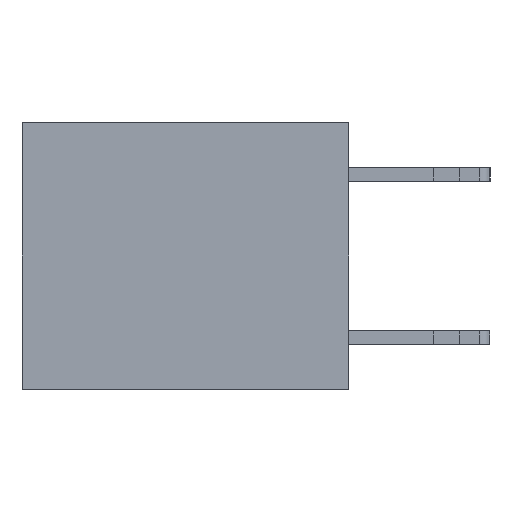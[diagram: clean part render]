
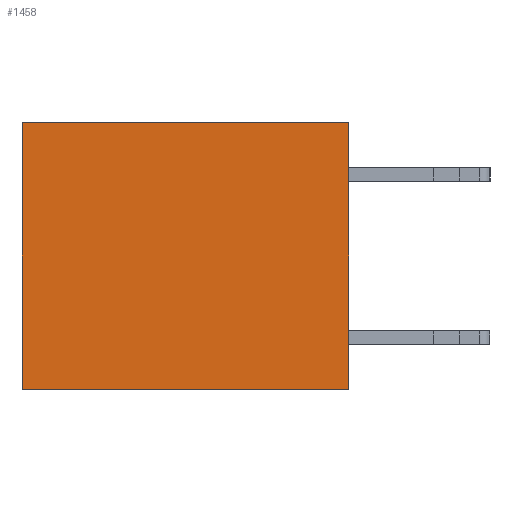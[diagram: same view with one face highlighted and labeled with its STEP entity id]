
A CAD part, left-side view. The second image highlights one B-rep face of the part: STEP entity #1458.
In plain terms, the highlighted planar face has unit normal (-1, 0, 0).
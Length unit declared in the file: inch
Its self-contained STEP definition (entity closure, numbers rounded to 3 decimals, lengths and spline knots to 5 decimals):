
#88 = ORIENTED_EDGE ( 'NONE', *, *, #11101, .T. ) ;
#96 = LINE ( 'NONE', #9933, #14800 ) ;
#450 = CARTESIAN_POINT ( 'NONE',  ( 0.3165, 0., 0. ) ) ;
#704 = VERTEX_POINT ( 'NONE', #18247 ) ;
#1458 = ADVANCED_FACE ( 'NONE', ( #15243 ), #18003, .F. ) ;
#2218 = AXIS2_PLACEMENT_3D ( 'NONE', #15051, #9306, #4893 ) ;
#3827 = LINE ( 'NONE', #7622, #7170 ) ;
#4893 = DIRECTION ( 'NONE',  ( 0., 0., -1. ) ) ;
#4894 = CARTESIAN_POINT ( 'NONE',  ( 0.3165, 0., -0.49 ) ) ;
#5191 = VERTEX_POINT ( 'NONE', #5452 ) ;
#5337 = EDGE_CURVE ( 'NONE', #12923, #704, #9621, .T. ) ;
#5452 = CARTESIAN_POINT ( 'NONE',  ( 0.3165, 0., -0.49 ) ) ;
#7170 = VECTOR ( 'NONE', #17742, 39.37008 ) ;
#7622 = CARTESIAN_POINT ( 'NONE',  ( 0.3165, 0., -0.49 ) ) ;
#7846 = ORIENTED_EDGE ( 'NONE', *, *, #13247, .F. ) ;
#8330 = EDGE_CURVE ( 'NONE', #5191, #14550, #11269, .T. ) ;
#9306 = DIRECTION ( 'NONE',  ( 1., 0., 0. ) ) ;
#9621 = LINE ( 'NONE', #12987, #15422 ) ;
#9926 = DIRECTION ( 'NONE',  ( 0., 1., 0. ) ) ;
#9933 = CARTESIAN_POINT ( 'NONE',  ( 0.3165, 0.6, -0.49 ) ) ;
#10321 = DIRECTION ( 'NONE',  ( 0., 1., 0. ) ) ;
#11101 = EDGE_CURVE ( 'NONE', #704, #14550, #96, .T. ) ;
#11269 = LINE ( 'NONE', #4894, #17119 ) ;
#11823 = ORIENTED_EDGE ( 'NONE', *, *, #8330, .F. ) ;
#11863 = CARTESIAN_POINT ( 'NONE',  ( 0.3165, 0.6, -0.49 ) ) ;
#12923 = VERTEX_POINT ( 'NONE', #450 ) ;
#12987 = CARTESIAN_POINT ( 'NONE',  ( 0.3165, 0., 0. ) ) ;
#13220 = EDGE_LOOP ( 'NONE', ( #88, #11823, #7846, #14473 ) ) ;
#13247 = EDGE_CURVE ( 'NONE', #12923, #5191, #3827, .T. ) ;
#14473 = ORIENTED_EDGE ( 'NONE', *, *, #5337, .T. ) ;
#14550 = VERTEX_POINT ( 'NONE', #11863 ) ;
#14800 = VECTOR ( 'NONE', #16294, 39.37008 ) ;
#15051 = CARTESIAN_POINT ( 'NONE',  ( 0.3165, 0., -0.49 ) ) ;
#15243 = FACE_OUTER_BOUND ( 'NONE', #13220, .T. ) ;
#15422 = VECTOR ( 'NONE', #9926, 39.37008 ) ;
#16294 = DIRECTION ( 'NONE',  ( 0., 0., -1. ) ) ;
#17119 = VECTOR ( 'NONE', #10321, 39.37008 ) ;
#17742 = DIRECTION ( 'NONE',  ( 0., 0., -1. ) ) ;
#18003 = PLANE ( 'NONE',  #2218 ) ;
#18247 = CARTESIAN_POINT ( 'NONE',  ( 0.3165, 0.6, 0. ) ) ;
